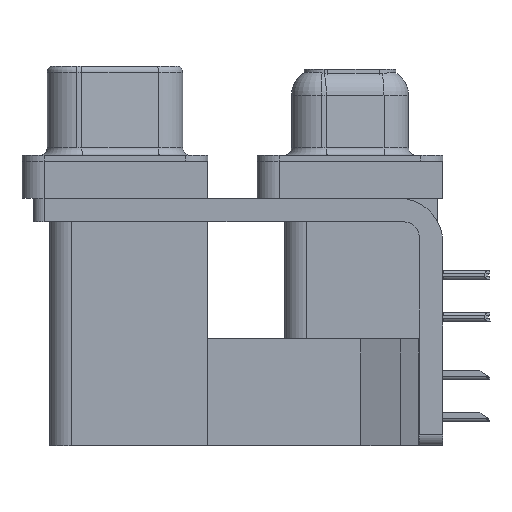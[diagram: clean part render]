
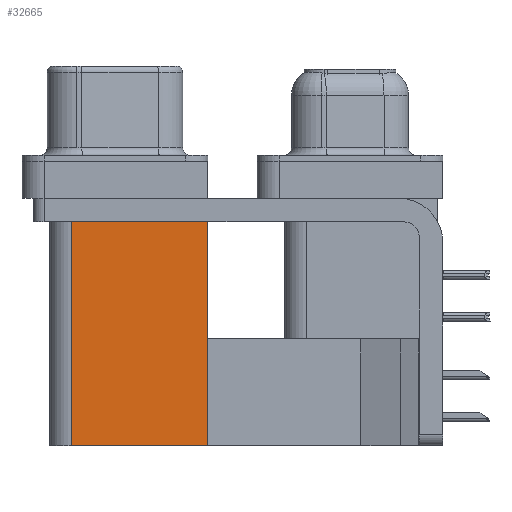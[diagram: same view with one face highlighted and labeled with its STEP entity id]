
A CAD part, left-side view. The second image highlights one B-rep face of the part: STEP entity #32665.
In plain terms, the highlighted planar face has unit normal (-1, 0, 0).
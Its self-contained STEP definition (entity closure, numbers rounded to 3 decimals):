
#660 = CARTESIAN_POINT ( 'NONE',  ( 3.79, 9.6, -19.2 ) ) ;
#1457 = VECTOR ( 'NONE', #4953, 1000. ) ;
#1841 = VERTEX_POINT ( 'NONE', #34886 ) ;
#4953 = DIRECTION ( 'NONE',  ( 0., 1., 0. ) ) ;
#5213 = ORIENTED_EDGE ( 'NONE', *, *, #6116, .F. ) ;
#6116 = EDGE_CURVE ( 'NONE', #29659, #15785, #16084, .T. ) ;
#6142 = LINE ( 'NONE', #20472, #30811 ) ;
#7825 = EDGE_CURVE ( 'NONE', #1841, #11969, #35551, .T. ) ;
#8593 = DIRECTION ( 'NONE',  ( 0., 0., -1. ) ) ;
#9141 = DIRECTION ( 'NONE',  ( 0., 0., 1. ) ) ;
#11061 = PLANE ( 'NONE',  #16694 ) ;
#11616 = DIRECTION ( 'NONE',  ( 1., 0., 0. ) ) ;
#11969 = VERTEX_POINT ( 'NONE', #35895 ) ;
#12315 = LINE ( 'NONE', #14781, #33405 ) ;
#12885 = DIRECTION ( 'NONE',  ( 0., 1., 0. ) ) ;
#14150 = EDGE_LOOP ( 'NONE', ( #16034, #36548, #5213, #25079 ) ) ;
#14781 = CARTESIAN_POINT ( 'NONE',  ( 3.79, 18.8, -19.2 ) ) ;
#15785 = VERTEX_POINT ( 'NONE', #25831 ) ;
#16034 = ORIENTED_EDGE ( 'NONE', *, *, #7825, .T. ) ;
#16084 = LINE ( 'NONE', #27950, #24853 ) ;
#16694 = AXIS2_PLACEMENT_3D ( 'NONE', #31216, #11616, #8593 ) ;
#17086 = FACE_OUTER_BOUND ( 'NONE', #14150, .T. ) ;
#20472 = CARTESIAN_POINT ( 'NONE',  ( 3.79, 9.6, -19.2 ) ) ;
#24853 = VECTOR ( 'NONE', #12885, 1000. ) ;
#25079 = ORIENTED_EDGE ( 'NONE', *, *, #25945, .T. ) ;
#25831 = CARTESIAN_POINT ( 'NONE',  ( 3.79, 18.8, -19.2 ) ) ;
#25892 = DIRECTION ( 'NONE',  ( 0., 0., 1. ) ) ;
#25945 = EDGE_CURVE ( 'NONE', #29659, #1841, #6142, .T. ) ;
#27950 = CARTESIAN_POINT ( 'NONE',  ( 3.79, 9.6, -19.2 ) ) ;
#29659 = VERTEX_POINT ( 'NONE', #660 ) ;
#30811 = VECTOR ( 'NONE', #9141, 1000. ) ;
#31216 = CARTESIAN_POINT ( 'NONE',  ( 3.79, 9.6, -19.2 ) ) ;
#32531 = CARTESIAN_POINT ( 'NONE',  ( 3.79, 9.6, -2.5 ) ) ;
#32665 = ADVANCED_FACE ( 'NONE', ( #17086 ), #11061, .F. ) ;
#33405 = VECTOR ( 'NONE', #25892, 1000. ) ;
#34886 = CARTESIAN_POINT ( 'NONE',  ( 3.79, 9.6, -2.5 ) ) ;
#35506 = EDGE_CURVE ( 'NONE', #15785, #11969, #12315, .T. ) ;
#35551 = LINE ( 'NONE', #32531, #1457 ) ;
#35895 = CARTESIAN_POINT ( 'NONE',  ( 3.79, 18.8, -2.5 ) ) ;
#36548 = ORIENTED_EDGE ( 'NONE', *, *, #35506, .F. ) ;
